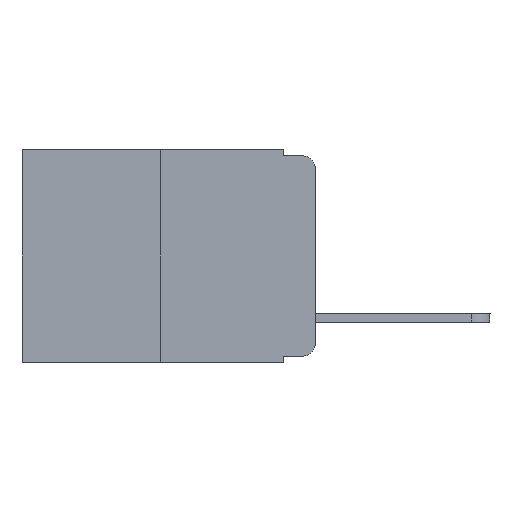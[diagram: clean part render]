
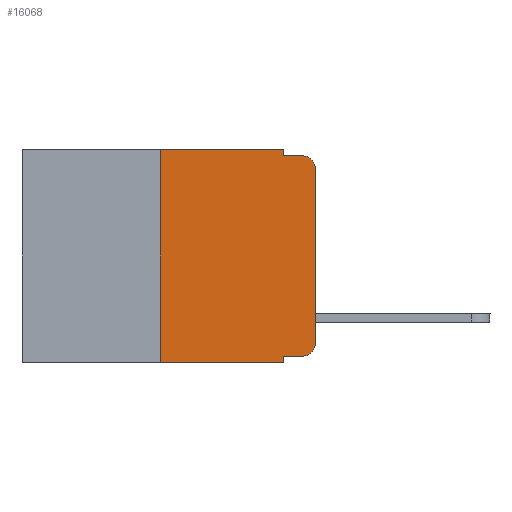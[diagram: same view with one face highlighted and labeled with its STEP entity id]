
A CAD part, left-side view. The second image highlights one B-rep face of the part: STEP entity #16068.
In plain terms, the highlighted planar face has unit normal (-1, 0, 0).
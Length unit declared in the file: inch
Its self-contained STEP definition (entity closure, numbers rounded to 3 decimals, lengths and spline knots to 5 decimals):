
#85 = DIRECTION ( 'NONE',  ( 0., 0., 1. ) ) ;
#199 = CARTESIAN_POINT ( 'NONE',  ( 0., 0.051, 0. ) ) ;
#674 = VECTOR ( 'NONE', #5061, 39.37008 ) ;
#685 = DIRECTION ( 'NONE',  ( 0., -1., 0. ) ) ;
#1338 = CARTESIAN_POINT ( 'NONE',  ( 0., 0.473, 0. ) ) ;
#1502 = VECTOR ( 'NONE', #15198, 39.37008 ) ;
#1546 = EDGE_CURVE ( 'NONE', #16730, #10512, #9337, .T. ) ;
#1706 = CARTESIAN_POINT ( 'NONE',  ( 0., 0.25, -0.343 ) ) ;
#1747 = EDGE_CURVE ( 'NONE', #16983, #2684, #1779, .T. ) ;
#1779 = LINE ( 'NONE', #12291, #15579 ) ;
#1815 = ORIENTED_EDGE ( 'NONE', *, *, #8294, .T. ) ;
#1939 = ORIENTED_EDGE ( 'NONE', *, *, #3284, .F. ) ;
#2115 = VECTOR ( 'NONE', #3736, 39.37008 ) ;
#2415 = VERTEX_POINT ( 'NONE', #5754 ) ;
#2519 = CARTESIAN_POINT ( 'NONE',  ( 0., 0.051, -0.333 ) ) ;
#2524 = LINE ( 'NONE', #5829, #1502 ) ;
#2560 = LINE ( 'NONE', #14478, #674 ) ;
#2622 = CIRCLE ( 'NONE', #9487, 0.02 ) ;
#2684 = VERTEX_POINT ( 'NONE', #8828 ) ;
#3021 = EDGE_LOOP ( 'NONE', ( #16993, #1815, #1939, #13524, #3890, #9365, #17270, #8697, #13012, #4242 ) ) ;
#3284 = EDGE_CURVE ( 'NONE', #10512, #5510, #2560, .T. ) ;
#3736 = DIRECTION ( 'NONE',  ( 0., -1., 0. ) ) ;
#3861 = EDGE_CURVE ( 'NONE', #2415, #15019, #4614, .T. ) ;
#3890 = ORIENTED_EDGE ( 'NONE', *, *, #16994, .F. ) ;
#4242 = ORIENTED_EDGE ( 'NONE', *, *, #7331, .T. ) ;
#4361 = AXIS2_PLACEMENT_3D ( 'NONE', #1338, #5354, #5297 ) ;
#4461 = EDGE_CURVE ( 'NONE', #6917, #14139, #8585, .T. ) ;
#4614 = LINE ( 'NONE', #2519, #2115 ) ;
#4921 = DIRECTION ( 'NONE',  ( 0., 0., -1. ) ) ;
#5017 = VECTOR ( 'NONE', #685, 39.37008 ) ;
#5061 = DIRECTION ( 'NONE',  ( 0., -1., 0. ) ) ;
#5167 = CARTESIAN_POINT ( 'NONE',  ( 0., 0., -0.03 ) ) ;
#5297 = DIRECTION ( 'NONE',  ( 0., 0., -1. ) ) ;
#5354 = DIRECTION ( 'NONE',  ( 1., 0., 0. ) ) ;
#5510 = VERTEX_POINT ( 'NONE', #15960 ) ;
#5596 = CARTESIAN_POINT ( 'NONE',  ( 0., 0., 0. ) ) ;
#5644 = VECTOR ( 'NONE', #12527, 39.37008 ) ;
#5754 = CARTESIAN_POINT ( 'NONE',  ( 0., 0.051, -0.333 ) ) ;
#5829 = CARTESIAN_POINT ( 'NONE',  ( 0., 0.473, 0. ) ) ;
#5837 = LINE ( 'NONE', #5912, #5644 ) ;
#5912 = CARTESIAN_POINT ( 'NONE',  ( 0., 0.051, 0. ) ) ;
#6027 = DIRECTION ( 'NONE',  ( -1., 0., 0. ) ) ;
#6597 = CARTESIAN_POINT ( 'NONE',  ( 0., 0., -0.313 ) ) ;
#6917 = VERTEX_POINT ( 'NONE', #6597 ) ;
#7331 = EDGE_CURVE ( 'NONE', #15019, #6917, #2622, .T. ) ;
#7375 = VERTEX_POINT ( 'NONE', #9108 ) ;
#7646 = CARTESIAN_POINT ( 'NONE',  ( 0., 0.051, 0. ) ) ;
#7862 = VECTOR ( 'NONE', #9049, 39.37008 ) ;
#7973 = CIRCLE ( 'NONE', #16722, 0.02 ) ;
#8294 = EDGE_CURVE ( 'NONE', #14139, #5510, #7973, .T. ) ;
#8338 = EDGE_CURVE ( 'NONE', #2415, #7375, #5837, .T. ) ;
#8455 = CARTESIAN_POINT ( 'NONE',  ( 0., 0.02, -0.333 ) ) ;
#8585 = LINE ( 'NONE', #5596, #13395 ) ;
#8697 = ORIENTED_EDGE ( 'NONE', *, *, #8338, .F. ) ;
#8828 = CARTESIAN_POINT ( 'NONE',  ( 0., 0.25, 0. ) ) ;
#9049 = DIRECTION ( 'NONE',  ( 0., 0., -1. ) ) ;
#9108 = CARTESIAN_POINT ( 'NONE',  ( 0., 0.051, -0.343 ) ) ;
#9314 = PLANE ( 'NONE',  #4361 ) ;
#9337 = LINE ( 'NONE', #7646, #7862 ) ;
#9365 = ORIENTED_EDGE ( 'NONE', *, *, #1747, .F. ) ;
#9487 = AXIS2_PLACEMENT_3D ( 'NONE', #11591, #12932, #4921 ) ;
#9720 = DIRECTION ( 'NONE',  ( 0., 0., 1. ) ) ;
#10123 = CARTESIAN_POINT ( 'NONE',  ( 0., 0.473, -0.343 ) ) ;
#10512 = VERTEX_POINT ( 'NONE', #13632 ) ;
#11288 = LINE ( 'NONE', #10123, #5017 ) ;
#11591 = CARTESIAN_POINT ( 'NONE',  ( 0., 0.02, -0.313 ) ) ;
#12291 = CARTESIAN_POINT ( 'NONE',  ( 0., 0.25, 0. ) ) ;
#12527 = DIRECTION ( 'NONE',  ( 0., 0., -1. ) ) ;
#12932 = DIRECTION ( 'NONE',  ( -1., 0., 0. ) ) ;
#13012 = ORIENTED_EDGE ( 'NONE', *, *, #3861, .T. ) ;
#13395 = VECTOR ( 'NONE', #9720, 39.37008 ) ;
#13524 = ORIENTED_EDGE ( 'NONE', *, *, #1546, .F. ) ;
#13632 = CARTESIAN_POINT ( 'NONE',  ( 0., 0.051, -0.01 ) ) ;
#14139 = VERTEX_POINT ( 'NONE', #5167 ) ;
#14478 = CARTESIAN_POINT ( 'NONE',  ( 0., 0.051, -0.01 ) ) ;
#15019 = VERTEX_POINT ( 'NONE', #8455 ) ;
#15155 = CARTESIAN_POINT ( 'NONE',  ( 0., 0.02, -0.03 ) ) ;
#15198 = DIRECTION ( 'NONE',  ( 0., -1., 0. ) ) ;
#15579 = VECTOR ( 'NONE', #85, 39.37008 ) ;
#15681 = FACE_OUTER_BOUND ( 'NONE', #3021, .T. ) ;
#15752 = EDGE_CURVE ( 'NONE', #16983, #7375, #11288, .T. ) ;
#15960 = CARTESIAN_POINT ( 'NONE',  ( 0., 0.02, -0.01 ) ) ;
#16068 = ADVANCED_FACE ( 'NONE', ( #15681 ), #9314, .F. ) ;
#16712 = DIRECTION ( 'NONE',  ( 0., 0., -1. ) ) ;
#16722 = AXIS2_PLACEMENT_3D ( 'NONE', #15155, #6027, #16712 ) ;
#16730 = VERTEX_POINT ( 'NONE', #199 ) ;
#16983 = VERTEX_POINT ( 'NONE', #1706 ) ;
#16993 = ORIENTED_EDGE ( 'NONE', *, *, #4461, .T. ) ;
#16994 = EDGE_CURVE ( 'NONE', #2684, #16730, #2524, .T. ) ;
#17270 = ORIENTED_EDGE ( 'NONE', *, *, #15752, .T. ) ;
